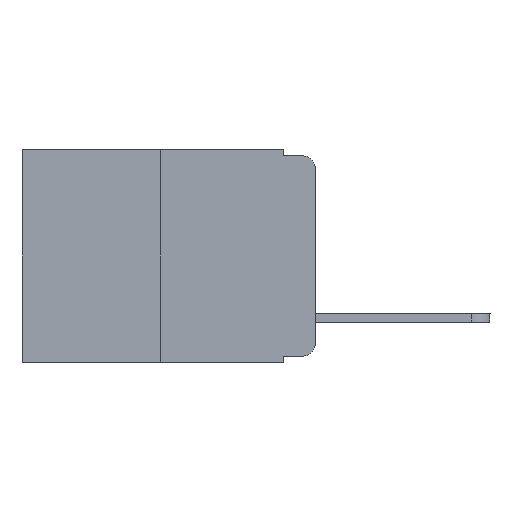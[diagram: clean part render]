
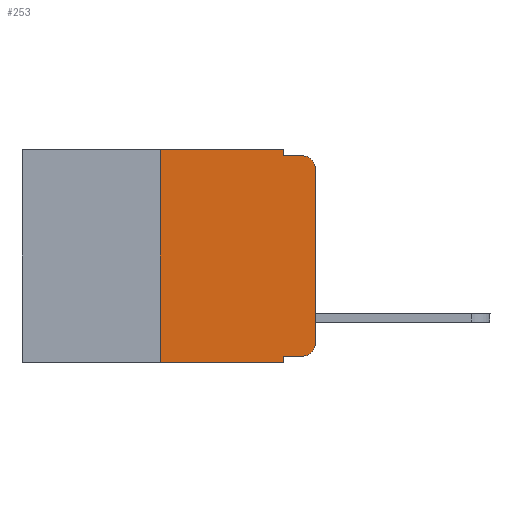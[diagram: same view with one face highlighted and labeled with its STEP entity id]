
A CAD part, left-side view. The second image highlights one B-rep face of the part: STEP entity #253.
In plain terms, the highlighted planar face has unit normal (-1, 0, 0).
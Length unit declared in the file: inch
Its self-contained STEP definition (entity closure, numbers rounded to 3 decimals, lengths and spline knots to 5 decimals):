
#145 = ORIENTED_EDGE ( 'NONE', *, *, #8064, .T. ) ;
#253 = ADVANCED_FACE ( 'NONE', ( #4193 ), #13879, .F. ) ;
#275 = ORIENTED_EDGE ( 'NONE', *, *, #5888, .T. ) ;
#347 = VERTEX_POINT ( 'NONE', #4336 ) ;
#375 = DIRECTION ( 'NONE',  ( 0., 0., -1. ) ) ;
#480 = CARTESIAN_POINT ( 'NONE',  ( 0., 0.25, 0. ) ) ;
#869 = DIRECTION ( 'NONE',  ( 0., 0., -1. ) ) ;
#911 = LINE ( 'NONE', #13020, #7181 ) ;
#1503 = ORIENTED_EDGE ( 'NONE', *, *, #10849, .F. ) ;
#1505 = ORIENTED_EDGE ( 'NONE', *, *, #9600, .F. ) ;
#1549 = DIRECTION ( 'NONE',  ( -1., 0., 0. ) ) ;
#1665 = VECTOR ( 'NONE', #12495, 39.37008 ) ;
#1714 = DIRECTION ( 'NONE',  ( 0., 0., -1. ) ) ;
#1740 = CIRCLE ( 'NONE', #7763, 0.02 ) ;
#1787 = ORIENTED_EDGE ( 'NONE', *, *, #11507, .T. ) ;
#1868 = DIRECTION ( 'NONE',  ( 1., 0., 0. ) ) ;
#1905 = VERTEX_POINT ( 'NONE', #9252 ) ;
#2019 = CARTESIAN_POINT ( 'NONE',  ( 0., 0.02, -0.333 ) ) ;
#2200 = LINE ( 'NONE', #14205, #14409 ) ;
#2344 = CARTESIAN_POINT ( 'NONE',  ( 0., 0.473, 0. ) ) ;
#2685 = DIRECTION ( 'NONE',  ( 0., 0., -1. ) ) ;
#2744 = CARTESIAN_POINT ( 'NONE',  ( 0., 0.473, 0. ) ) ;
#2938 = ORIENTED_EDGE ( 'NONE', *, *, #5211, .F. ) ;
#3376 = VERTEX_POINT ( 'NONE', #4331 ) ;
#3568 = ORIENTED_EDGE ( 'NONE', *, *, #10404, .F. ) ;
#3977 = DIRECTION ( 'NONE',  ( 0., -1., 0. ) ) ;
#4193 = FACE_OUTER_BOUND ( 'NONE', #6173, .T. ) ;
#4309 = DIRECTION ( 'NONE',  ( 0., 0., 1. ) ) ;
#4331 = CARTESIAN_POINT ( 'NONE',  ( 0., 0.051, -0.01 ) ) ;
#4336 = CARTESIAN_POINT ( 'NONE',  ( 0., 0., -0.03 ) ) ;
#4344 = CARTESIAN_POINT ( 'NONE',  ( 0., 0.051, 0. ) ) ;
#5053 = LINE ( 'NONE', #13938, #11649 ) ;
#5211 = EDGE_CURVE ( 'NONE', #12243, #8659, #8862, .T. ) ;
#5321 = DIRECTION ( 'NONE',  ( 0., -1., 0. ) ) ;
#5810 = VECTOR ( 'NONE', #10565, 39.37008 ) ;
#5888 = EDGE_CURVE ( 'NONE', #7369, #6560, #1740, .T. ) ;
#6173 = EDGE_LOOP ( 'NONE', ( #145, #12227, #1503, #1505, #2938, #7781, #1787, #3568, #6198, #275 ) ) ;
#6198 = ORIENTED_EDGE ( 'NONE', *, *, #13940, .T. ) ;
#6560 = VERTEX_POINT ( 'NONE', #12373 ) ;
#6609 = DIRECTION ( 'NONE',  ( 0., -1., 0. ) ) ;
#7082 = CARTESIAN_POINT ( 'NONE',  ( 0., 0.02, -0.03 ) ) ;
#7135 = VECTOR ( 'NONE', #4309, 39.37008 ) ;
#7144 = LINE ( 'NONE', #8252, #5810 ) ;
#7161 = LINE ( 'NONE', #12577, #1665 ) ;
#7181 = VECTOR ( 'NONE', #11769, 39.37008 ) ;
#7369 = VERTEX_POINT ( 'NONE', #2019 ) ;
#7504 = LINE ( 'NONE', #10830, #9019 ) ;
#7638 = CARTESIAN_POINT ( 'NONE',  ( 0., 0., 0. ) ) ;
#7763 = AXIS2_PLACEMENT_3D ( 'NONE', #11627, #13822, #2685 ) ;
#7781 = ORIENTED_EDGE ( 'NONE', *, *, #11365, .F. ) ;
#7810 = CARTESIAN_POINT ( 'NONE',  ( 0., 0.02, -0.01 ) ) ;
#7871 = VERTEX_POINT ( 'NONE', #7810 ) ;
#8064 = EDGE_CURVE ( 'NONE', #6560, #347, #13124, .T. ) ;
#8252 = CARTESIAN_POINT ( 'NONE',  ( 0., 0.25, 0. ) ) ;
#8632 = AXIS2_PLACEMENT_3D ( 'NONE', #7082, #1549, #375 ) ;
#8659 = VERTEX_POINT ( 'NONE', #4344 ) ;
#8862 = LINE ( 'NONE', #2344, #12072 ) ;
#9019 = VECTOR ( 'NONE', #869, 39.37008 ) ;
#9097 = CIRCLE ( 'NONE', #8632, 0.02 ) ;
#9252 = CARTESIAN_POINT ( 'NONE',  ( 0., 0.051, -0.333 ) ) ;
#9574 = AXIS2_PLACEMENT_3D ( 'NONE', #2744, #1868, #1714 ) ;
#9600 = EDGE_CURVE ( 'NONE', #8659, #3376, #7504, .T. ) ;
#10404 = EDGE_CURVE ( 'NONE', #1905, #12317, #911, .T. ) ;
#10565 = DIRECTION ( 'NONE',  ( 0., 0., 1. ) ) ;
#10830 = CARTESIAN_POINT ( 'NONE',  ( 0., 0.051, 0. ) ) ;
#10849 = EDGE_CURVE ( 'NONE', #3376, #7871, #2200, .T. ) ;
#10906 = VERTEX_POINT ( 'NONE', #11052 ) ;
#11052 = CARTESIAN_POINT ( 'NONE',  ( 0., 0.25, -0.343 ) ) ;
#11365 = EDGE_CURVE ( 'NONE', #10906, #12243, #7144, .T. ) ;
#11507 = EDGE_CURVE ( 'NONE', #10906, #12317, #5053, .T. ) ;
#11558 = CARTESIAN_POINT ( 'NONE',  ( 0., 0.051, -0.343 ) ) ;
#11627 = CARTESIAN_POINT ( 'NONE',  ( 0., 0.02, -0.313 ) ) ;
#11649 = VECTOR ( 'NONE', #3977, 39.37008 ) ;
#11769 = DIRECTION ( 'NONE',  ( 0., 0., -1. ) ) ;
#12072 = VECTOR ( 'NONE', #6609, 39.37008 ) ;
#12227 = ORIENTED_EDGE ( 'NONE', *, *, #14430, .T. ) ;
#12243 = VERTEX_POINT ( 'NONE', #480 ) ;
#12317 = VERTEX_POINT ( 'NONE', #11558 ) ;
#12373 = CARTESIAN_POINT ( 'NONE',  ( 0., 0., -0.313 ) ) ;
#12495 = DIRECTION ( 'NONE',  ( 0., -1., 0. ) ) ;
#12577 = CARTESIAN_POINT ( 'NONE',  ( 0., 0.051, -0.333 ) ) ;
#13020 = CARTESIAN_POINT ( 'NONE',  ( 0., 0.051, 0. ) ) ;
#13124 = LINE ( 'NONE', #7638, #7135 ) ;
#13822 = DIRECTION ( 'NONE',  ( -1., 0., 0. ) ) ;
#13879 = PLANE ( 'NONE',  #9574 ) ;
#13938 = CARTESIAN_POINT ( 'NONE',  ( 0., 0.473, -0.343 ) ) ;
#13940 = EDGE_CURVE ( 'NONE', #1905, #7369, #7161, .T. ) ;
#14205 = CARTESIAN_POINT ( 'NONE',  ( 0., 0.051, -0.01 ) ) ;
#14409 = VECTOR ( 'NONE', #5321, 39.37008 ) ;
#14430 = EDGE_CURVE ( 'NONE', #347, #7871, #9097, .T. ) ;
